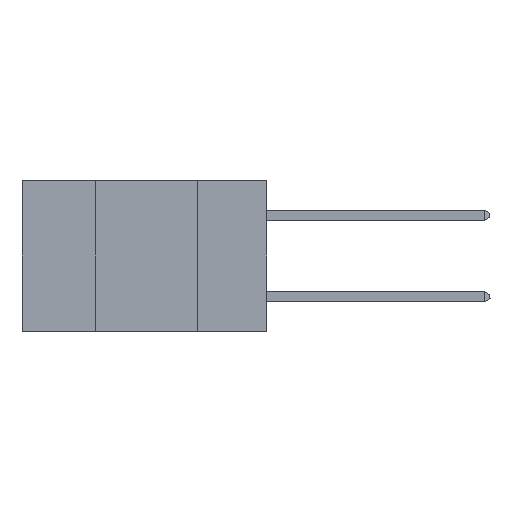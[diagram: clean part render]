
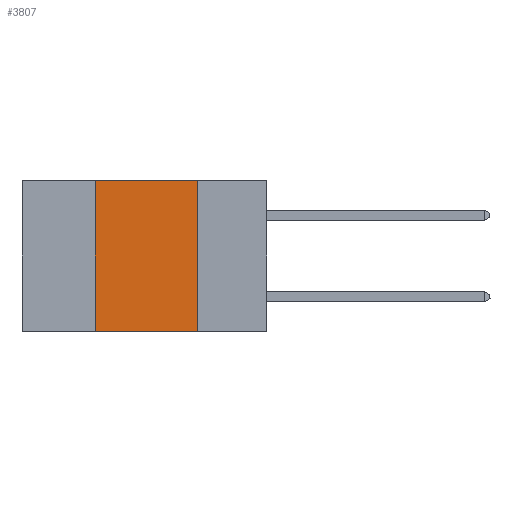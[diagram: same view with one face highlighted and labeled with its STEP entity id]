
A CAD part, left-side view. The second image highlights one B-rep face of the part: STEP entity #3807.
In plain terms, the highlighted planar face has unit normal (-1, 0, 0).
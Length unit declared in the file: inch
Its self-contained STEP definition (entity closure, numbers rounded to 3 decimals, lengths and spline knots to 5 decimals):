
#113 = DIRECTION ( 'NONE',  ( 0., 0., -1. ) ) ;
#511 = CARTESIAN_POINT ( 'NONE',  ( 0., 0.6, -0.37 ) ) ;
#1387 = VERTEX_POINT ( 'NONE', #6775 ) ;
#1473 = EDGE_CURVE ( 'NONE', #1481, #4406, #3459, .T. ) ;
#1481 = VERTEX_POINT ( 'NONE', #2955 ) ;
#1545 = LINE ( 'NONE', #8207, #1985 ) ;
#1923 = VECTOR ( 'NONE', #5379, 39.37008 ) ;
#1940 = CARTESIAN_POINT ( 'NONE',  ( 0., 0.6, 0. ) ) ;
#1985 = VECTOR ( 'NONE', #2539, 39.37008 ) ;
#2461 = EDGE_CURVE ( 'NONE', #4406, #4218, #9507, .T. ) ;
#2539 = DIRECTION ( 'NONE',  ( 0., 0., -1. ) ) ;
#2829 = PLANE ( 'NONE',  #4031 ) ;
#2955 = CARTESIAN_POINT ( 'NONE',  ( 0., 0.42, -0.37 ) ) ;
#3459 = LINE ( 'NONE', #5774, #11322 ) ;
#3807 = ADVANCED_FACE ( 'NONE', ( #5351 ), #2829, .F. ) ;
#4031 = AXIS2_PLACEMENT_3D ( 'NONE', #1940, #9420, #113 ) ;
#4144 = EDGE_LOOP ( 'NONE', ( #10709, #5504, #7516, #10847 ) ) ;
#4218 = VERTEX_POINT ( 'NONE', #4247 ) ;
#4247 = CARTESIAN_POINT ( 'NONE',  ( 0., 0.17, 0. ) ) ;
#4406 = VERTEX_POINT ( 'NONE', #10258 ) ;
#5028 = VECTOR ( 'NONE', #10843, 39.37008 ) ;
#5351 = FACE_OUTER_BOUND ( 'NONE', #4144, .T. ) ;
#5379 = DIRECTION ( 'NONE',  ( 0., -1., 0. ) ) ;
#5504 = ORIENTED_EDGE ( 'NONE', *, *, #2461, .F. ) ;
#5774 = CARTESIAN_POINT ( 'NONE',  ( 0., 0.42, 0. ) ) ;
#6335 = EDGE_CURVE ( 'NONE', #4218, #1387, #1545, .T. ) ;
#6775 = CARTESIAN_POINT ( 'NONE',  ( 0., 0.17, -0.37 ) ) ;
#7516 = ORIENTED_EDGE ( 'NONE', *, *, #1473, .F. ) ;
#8157 = EDGE_CURVE ( 'NONE', #1481, #1387, #10060, .T. ) ;
#8207 = CARTESIAN_POINT ( 'NONE',  ( 0., 0.17, 0. ) ) ;
#9420 = DIRECTION ( 'NONE',  ( 1., 0., 0. ) ) ;
#9507 = LINE ( 'NONE', #10922, #1923 ) ;
#10060 = LINE ( 'NONE', #511, #5028 ) ;
#10258 = CARTESIAN_POINT ( 'NONE',  ( 0., 0.42, 0. ) ) ;
#10709 = ORIENTED_EDGE ( 'NONE', *, *, #6335, .F. ) ;
#10843 = DIRECTION ( 'NONE',  ( 0., -1., 0. ) ) ;
#10847 = ORIENTED_EDGE ( 'NONE', *, *, #8157, .T. ) ;
#10922 = CARTESIAN_POINT ( 'NONE',  ( 0., 0.6, 0. ) ) ;
#11322 = VECTOR ( 'NONE', #11622, 39.37008 ) ;
#11622 = DIRECTION ( 'NONE',  ( 0., 0., 1. ) ) ;
